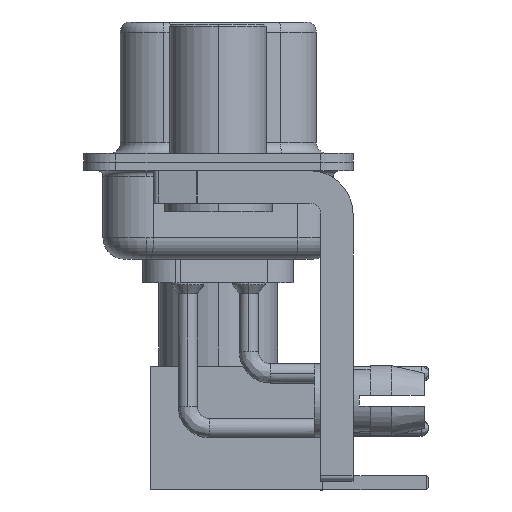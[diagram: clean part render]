
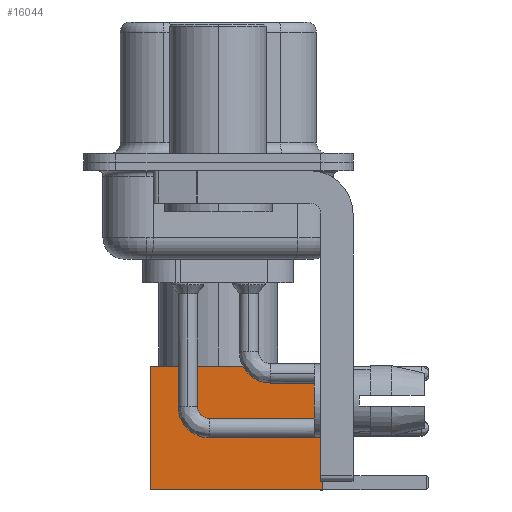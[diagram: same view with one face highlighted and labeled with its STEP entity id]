
A CAD part, left-side view. The second image highlights one B-rep face of the part: STEP entity #16044.
In plain terms, the highlighted face is planar.
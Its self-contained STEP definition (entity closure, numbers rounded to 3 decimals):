
#320 = DIRECTION ( 'NONE',  ( 0., 1., 0. ) ) ;
#503 = LINE ( 'NONE', #2481, #26728 ) ;
#1260 = ORIENTED_EDGE ( 'NONE', *, *, #22731, .T. ) ;
#2351 = ORIENTED_EDGE ( 'NONE', *, *, #16153, .F. ) ;
#2481 = CARTESIAN_POINT ( 'NONE',  ( 2.875, 2.875, 0. ) ) ;
#2592 = VERTEX_POINT ( 'NONE', #14502 ) ;
#3568 = AXIS2_PLACEMENT_3D ( 'NONE', #9078, #320, #4533 ) ;
#3712 = VERTEX_POINT ( 'NONE', #19256 ) ;
#4533 = DIRECTION ( 'NONE',  ( 0., 0., 1. ) ) ;
#5016 = DIRECTION ( 'NONE',  ( 0., 0., -1. ) ) ;
#5607 = LINE ( 'NONE', #14842, #21274 ) ;
#6624 = VERTEX_POINT ( 'NONE', #21301 ) ;
#6640 = CARTESIAN_POINT ( 'NONE',  ( 2.875, 2.875, 0. ) ) ;
#7697 = LINE ( 'NONE', #26140, #23374 ) ;
#9078 = CARTESIAN_POINT ( 'NONE',  ( 2.875, 2.875, 0. ) ) ;
#12698 = EDGE_CURVE ( 'NONE', #3712, #2592, #5607, .T. ) ;
#13407 = ORIENTED_EDGE ( 'NONE', *, *, #29731, .T. ) ;
#14502 = CARTESIAN_POINT ( 'NONE',  ( -2.875, 2.875, 0. ) ) ;
#14842 = CARTESIAN_POINT ( 'NONE',  ( -2.875, 2.875, 0. ) ) ;
#15333 = DIRECTION ( 'NONE',  ( -1., 0., 0. ) ) ;
#16044 = ADVANCED_FACE ( 'NONE', ( #18448 ), #27978, .T. ) ;
#16153 = EDGE_CURVE ( 'NONE', #6624, #3712, #7697, .T. ) ;
#18448 = FACE_OUTER_BOUND ( 'NONE', #18904, .T. ) ;
#18904 = EDGE_LOOP ( 'NONE', ( #13407, #1260, #19472, #2351 ) ) ;
#19256 = CARTESIAN_POINT ( 'NONE',  ( -2.875, 2.875, 8. ) ) ;
#19472 = ORIENTED_EDGE ( 'NONE', *, *, #12698, .F. ) ;
#21274 = VECTOR ( 'NONE', #24050, 1000. ) ;
#21301 = CARTESIAN_POINT ( 'NONE',  ( 2.875, 2.875, 8. ) ) ;
#22519 = VECTOR ( 'NONE', #15333, 1000. ) ;
#22731 = EDGE_CURVE ( 'NONE', #28877, #2592, #27264, .T. ) ;
#23374 = VECTOR ( 'NONE', #24164, 1000. ) ;
#24050 = DIRECTION ( 'NONE',  ( 0., 0., -1. ) ) ;
#24164 = DIRECTION ( 'NONE',  ( -1., 0., 0. ) ) ;
#26140 = CARTESIAN_POINT ( 'NONE',  ( 0., 2.875, 8. ) ) ;
#26728 = VECTOR ( 'NONE', #5016, 1000. ) ;
#27108 = CARTESIAN_POINT ( 'NONE',  ( 0., 2.875, 0. ) ) ;
#27264 = LINE ( 'NONE', #27108, #22519 ) ;
#27978 = PLANE ( 'NONE',  #3568 ) ;
#28877 = VERTEX_POINT ( 'NONE', #6640 ) ;
#29731 = EDGE_CURVE ( 'NONE', #6624, #28877, #503, .T. ) ;
